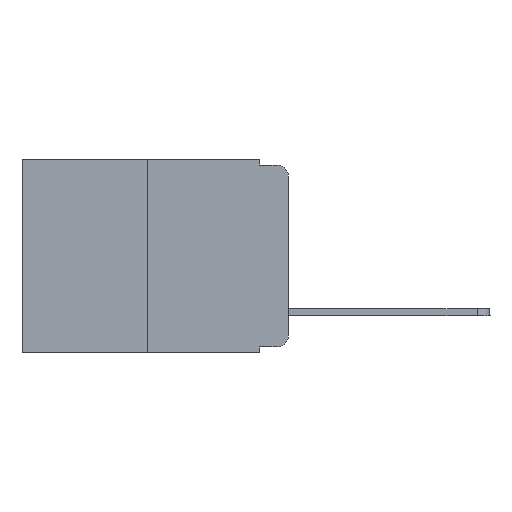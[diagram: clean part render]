
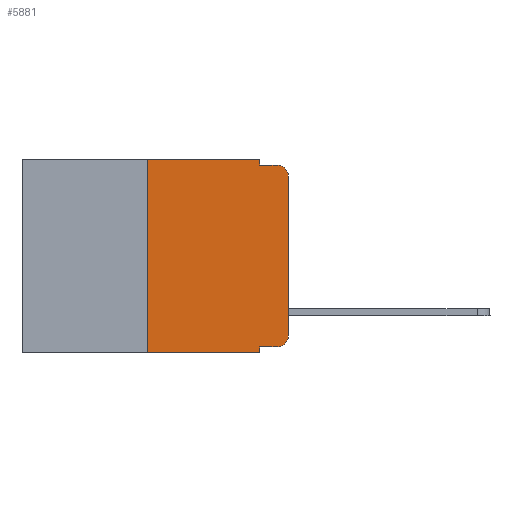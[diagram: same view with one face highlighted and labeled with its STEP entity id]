
A CAD part, left-side view. The second image highlights one B-rep face of the part: STEP entity #5881.
In plain terms, the highlighted planar face has unit normal (-1, 0, 0).
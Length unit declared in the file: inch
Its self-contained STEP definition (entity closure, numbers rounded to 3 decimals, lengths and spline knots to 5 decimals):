
#86 = DIRECTION ( 'NONE',  ( 0., 0., 1. ) ) ;
#174 = EDGE_CURVE ( 'NONE', #7820, #6242, #7062, .T. ) ;
#176 = VECTOR ( 'NONE', #3614, 39.37008 ) ;
#211 = ORIENTED_EDGE ( 'NONE', *, *, #9094, .T. ) ;
#322 = LINE ( 'NONE', #4959, #455 ) ;
#376 = EDGE_LOOP ( 'NONE', ( #9027, #7422, #3316, #3753, #8616, #1041, #4122, #6595, #9369, #211 ) ) ;
#455 = VECTOR ( 'NONE', #9759, 39.37008 ) ;
#555 = CARTESIAN_POINT ( 'NONE',  ( 0., 0.473, 0. ) ) ;
#613 = CARTESIAN_POINT ( 'NONE',  ( 0., 0.02, -0.03 ) ) ;
#733 = VECTOR ( 'NONE', #9634, 39.37008 ) ;
#745 = CIRCLE ( 'NONE', #6205, 0.02 ) ;
#1041 = ORIENTED_EDGE ( 'NONE', *, *, #174, .F. ) ;
#1207 = CARTESIAN_POINT ( 'NONE',  ( 0., 0.25, -0.343 ) ) ;
#1316 = DIRECTION ( 'NONE',  ( 0., -1., 0. ) ) ;
#1475 = DIRECTION ( 'NONE',  ( 1., 0., 0. ) ) ;
#1874 = VERTEX_POINT ( 'NONE', #8060 ) ;
#1944 = VERTEX_POINT ( 'NONE', #4304 ) ;
#2103 = EDGE_CURVE ( 'NONE', #4803, #3637, #5137, .T. ) ;
#2173 = DIRECTION ( 'NONE',  ( 0., 0., -1. ) ) ;
#2225 = DIRECTION ( 'NONE',  ( 0., 0., -1. ) ) ;
#2377 = CARTESIAN_POINT ( 'NONE',  ( 0., 0., -0.03 ) ) ;
#2552 = EDGE_CURVE ( 'NONE', #7820, #3756, #3213, .T. ) ;
#2737 = CARTESIAN_POINT ( 'NONE',  ( 0., 0.02, -0.313 ) ) ;
#2785 = LINE ( 'NONE', #7763, #4530 ) ;
#3213 = LINE ( 'NONE', #6515, #733 ) ;
#3316 = ORIENTED_EDGE ( 'NONE', *, *, #2103, .F. ) ;
#3464 = CIRCLE ( 'NONE', #3995, 0.02 ) ;
#3614 = DIRECTION ( 'NONE',  ( 0., 0., -1. ) ) ;
#3637 = VERTEX_POINT ( 'NONE', #10288 ) ;
#3751 = CARTESIAN_POINT ( 'NONE',  ( 0., 0., 0. ) ) ;
#3753 = ORIENTED_EDGE ( 'NONE', *, *, #9801, .F. ) ;
#3756 = VERTEX_POINT ( 'NONE', #6464 ) ;
#3978 = VERTEX_POINT ( 'NONE', #2377 ) ;
#3995 = AXIS2_PLACEMENT_3D ( 'NONE', #2737, #9191, #6747 ) ;
#4022 = CARTESIAN_POINT ( 'NONE',  ( 0., 0.25, 0. ) ) ;
#4122 = ORIENTED_EDGE ( 'NONE', *, *, #2552, .T. ) ;
#4304 = CARTESIAN_POINT ( 'NONE',  ( 0., 0.02, -0.333 ) ) ;
#4391 = CARTESIAN_POINT ( 'NONE',  ( 0., 0., -0.313 ) ) ;
#4530 = VECTOR ( 'NONE', #7083, 39.37008 ) ;
#4773 = DIRECTION ( 'NONE',  ( 0., -1., 0. ) ) ;
#4803 = VERTEX_POINT ( 'NONE', #10105 ) ;
#4843 = CARTESIAN_POINT ( 'NONE',  ( 0., 0.25, 0. ) ) ;
#4959 = CARTESIAN_POINT ( 'NONE',  ( 0., 0.051, 0. ) ) ;
#5085 = VERTEX_POINT ( 'NONE', #4391 ) ;
#5137 = LINE ( 'NONE', #8373, #7256 ) ;
#5218 = FACE_OUTER_BOUND ( 'NONE', #376, .T. ) ;
#5286 = VERTEX_POINT ( 'NONE', #8074 ) ;
#5326 = DIRECTION ( 'NONE',  ( 0., 0., 1. ) ) ;
#5792 = EDGE_CURVE ( 'NONE', #3978, #3637, #745, .T. ) ;
#5826 = VECTOR ( 'NONE', #86, 39.37008 ) ;
#5881 = ADVANCED_FACE ( 'NONE', ( #5218 ), #7559, .F. ) ;
#6205 = AXIS2_PLACEMENT_3D ( 'NONE', #613, #10069, #2173 ) ;
#6242 = VERTEX_POINT ( 'NONE', #4022 ) ;
#6464 = CARTESIAN_POINT ( 'NONE',  ( 0., 0.051, -0.343 ) ) ;
#6515 = CARTESIAN_POINT ( 'NONE',  ( 0., 0.473, -0.343 ) ) ;
#6544 = VECTOR ( 'NONE', #5326, 39.37008 ) ;
#6595 = ORIENTED_EDGE ( 'NONE', *, *, #8484, .F. ) ;
#6747 = DIRECTION ( 'NONE',  ( 0., 0., -1. ) ) ;
#7062 = LINE ( 'NONE', #4843, #5826 ) ;
#7083 = DIRECTION ( 'NONE',  ( 0., -1., 0. ) ) ;
#7256 = VECTOR ( 'NONE', #1316, 39.37008 ) ;
#7422 = ORIENTED_EDGE ( 'NONE', *, *, #5792, .T. ) ;
#7498 = EDGE_CURVE ( 'NONE', #5085, #3978, #8164, .T. ) ;
#7559 = PLANE ( 'NONE',  #7983 ) ;
#7763 = CARTESIAN_POINT ( 'NONE',  ( 0., 0.473, 0. ) ) ;
#7771 = VECTOR ( 'NONE', #4773, 39.37008 ) ;
#7820 = VERTEX_POINT ( 'NONE', #1207 ) ;
#7947 = EDGE_CURVE ( 'NONE', #6242, #5286, #2785, .T. ) ;
#7983 = AXIS2_PLACEMENT_3D ( 'NONE', #555, #1475, #2225 ) ;
#8060 = CARTESIAN_POINT ( 'NONE',  ( 0., 0.051, -0.333 ) ) ;
#8074 = CARTESIAN_POINT ( 'NONE',  ( 0., 0.051, 0. ) ) ;
#8164 = LINE ( 'NONE', #3751, #6544 ) ;
#8373 = CARTESIAN_POINT ( 'NONE',  ( 0., 0.051, -0.01 ) ) ;
#8475 = CARTESIAN_POINT ( 'NONE',  ( 0., 0.051, 0. ) ) ;
#8484 = EDGE_CURVE ( 'NONE', #1874, #3756, #9265, .T. ) ;
#8616 = ORIENTED_EDGE ( 'NONE', *, *, #7947, .F. ) ;
#8707 = EDGE_CURVE ( 'NONE', #1874, #1944, #9639, .T. ) ;
#9027 = ORIENTED_EDGE ( 'NONE', *, *, #7498, .T. ) ;
#9094 = EDGE_CURVE ( 'NONE', #1944, #5085, #3464, .T. ) ;
#9191 = DIRECTION ( 'NONE',  ( -1., 0., 0. ) ) ;
#9265 = LINE ( 'NONE', #8475, #176 ) ;
#9369 = ORIENTED_EDGE ( 'NONE', *, *, #8707, .T. ) ;
#9547 = CARTESIAN_POINT ( 'NONE',  ( 0., 0.051, -0.333 ) ) ;
#9634 = DIRECTION ( 'NONE',  ( 0., -1., 0. ) ) ;
#9639 = LINE ( 'NONE', #9547, #7771 ) ;
#9759 = DIRECTION ( 'NONE',  ( 0., 0., -1. ) ) ;
#9801 = EDGE_CURVE ( 'NONE', #5286, #4803, #322, .T. ) ;
#10069 = DIRECTION ( 'NONE',  ( -1., 0., 0. ) ) ;
#10105 = CARTESIAN_POINT ( 'NONE',  ( 0., 0.051, -0.01 ) ) ;
#10288 = CARTESIAN_POINT ( 'NONE',  ( 0., 0.02, -0.01 ) ) ;
